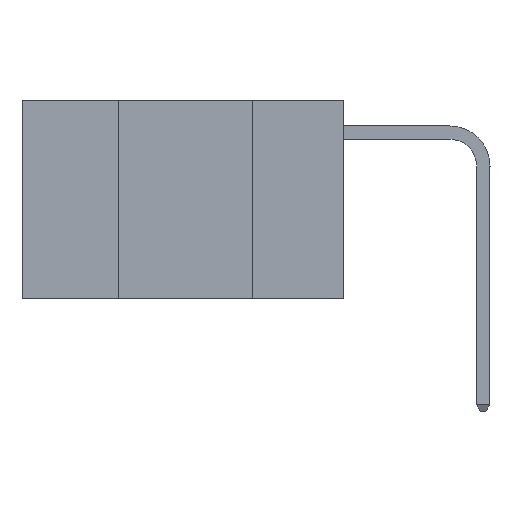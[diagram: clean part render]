
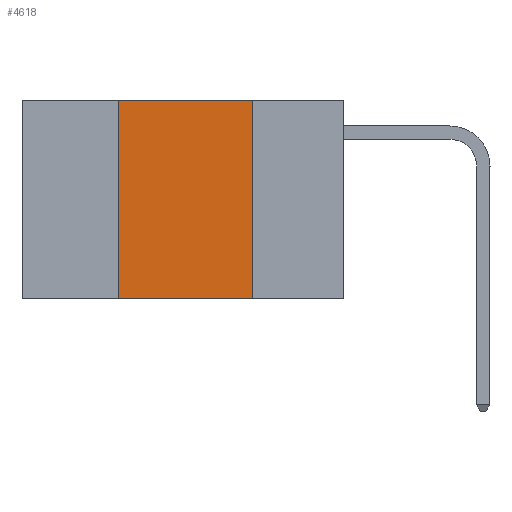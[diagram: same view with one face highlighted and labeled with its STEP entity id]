
A CAD part, left-side view. The second image highlights one B-rep face of the part: STEP entity #4618.
In plain terms, the highlighted planar face has unit normal (-1, 0, 0).
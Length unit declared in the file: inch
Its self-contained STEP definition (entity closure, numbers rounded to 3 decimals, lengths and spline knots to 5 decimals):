
#20 = LINE ( 'NONE', #8596, #12166 ) ;
#779 = VERTEX_POINT ( 'NONE', #2084 ) ;
#1401 = DIRECTION ( 'NONE',  ( 1., 0., 0. ) ) ;
#1441 = FACE_OUTER_BOUND ( 'NONE', #2522, .T. ) ;
#1865 = LINE ( 'NONE', #11888, #4185 ) ;
#1905 = LINE ( 'NONE', #6162, #11743 ) ;
#2084 = CARTESIAN_POINT ( 'NONE',  ( 0., 0.17, -0.37 ) ) ;
#2131 = CARTESIAN_POINT ( 'NONE',  ( 0., 0.42, 0. ) ) ;
#2522 = EDGE_LOOP ( 'NONE', ( #4451, #6991, #11956, #4749 ) ) ;
#2627 = CARTESIAN_POINT ( 'NONE',  ( 0., 0.42, -0.37 ) ) ;
#2871 = DIRECTION ( 'NONE',  ( 0., 0., 1. ) ) ;
#3602 = VERTEX_POINT ( 'NONE', #2627 ) ;
#4185 = VECTOR ( 'NONE', #7218, 39.37008 ) ;
#4345 = CARTESIAN_POINT ( 'NONE',  ( 0., 0.6, 0. ) ) ;
#4451 = ORIENTED_EDGE ( 'NONE', *, *, #7188, .F. ) ;
#4603 = CARTESIAN_POINT ( 'NONE',  ( 0., 0.6, -0.37 ) ) ;
#4618 = ADVANCED_FACE ( 'NONE', ( #1441 ), #10037, .F. ) ;
#4749 = ORIENTED_EDGE ( 'NONE', *, *, #9897, .T. ) ;
#5241 = EDGE_CURVE ( 'NONE', #10890, #8867, #1905, .T. ) ;
#6098 = AXIS2_PLACEMENT_3D ( 'NONE', #4345, #1401, #8169 ) ;
#6162 = CARTESIAN_POINT ( 'NONE',  ( 0., 0.6, 0. ) ) ;
#6991 = ORIENTED_EDGE ( 'NONE', *, *, #5241, .F. ) ;
#7188 = EDGE_CURVE ( 'NONE', #8867, #779, #1865, .T. ) ;
#7218 = DIRECTION ( 'NONE',  ( 0., 0., -1. ) ) ;
#7230 = LINE ( 'NONE', #4603, #9776 ) ;
#7421 = DIRECTION ( 'NONE',  ( 0., -1., 0. ) ) ;
#8169 = DIRECTION ( 'NONE',  ( 0., 0., -1. ) ) ;
#8596 = CARTESIAN_POINT ( 'NONE',  ( 0., 0.42, 0. ) ) ;
#8867 = VERTEX_POINT ( 'NONE', #10636 ) ;
#9776 = VECTOR ( 'NONE', #7421, 39.37008 ) ;
#9897 = EDGE_CURVE ( 'NONE', #3602, #779, #7230, .T. ) ;
#10037 = PLANE ( 'NONE',  #6098 ) ;
#10636 = CARTESIAN_POINT ( 'NONE',  ( 0., 0.17, 0. ) ) ;
#10890 = VERTEX_POINT ( 'NONE', #2131 ) ;
#11050 = EDGE_CURVE ( 'NONE', #3602, #10890, #20, .T. ) ;
#11743 = VECTOR ( 'NONE', #11813, 39.37008 ) ;
#11813 = DIRECTION ( 'NONE',  ( 0., -1., 0. ) ) ;
#11888 = CARTESIAN_POINT ( 'NONE',  ( 0., 0.17, 0. ) ) ;
#11956 = ORIENTED_EDGE ( 'NONE', *, *, #11050, .F. ) ;
#12166 = VECTOR ( 'NONE', #2871, 39.37008 ) ;
